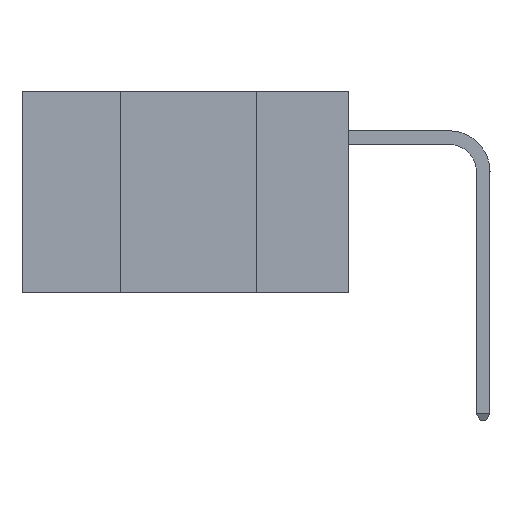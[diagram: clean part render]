
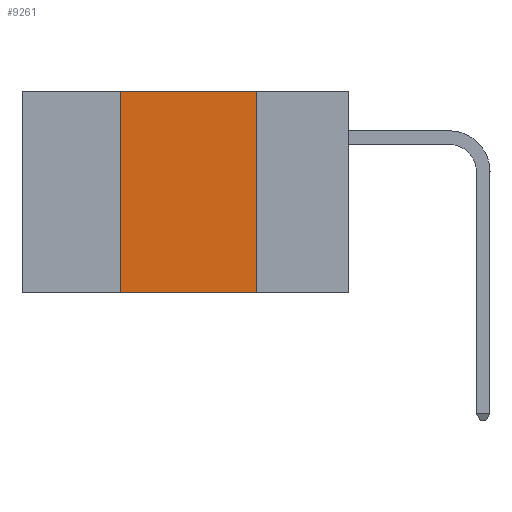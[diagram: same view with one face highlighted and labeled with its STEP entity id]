
A CAD part, left-side view. The second image highlights one B-rep face of the part: STEP entity #9261.
In plain terms, the highlighted planar face has unit normal (-1, 0, 0).
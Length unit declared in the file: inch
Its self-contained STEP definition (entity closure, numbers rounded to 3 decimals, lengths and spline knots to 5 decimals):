
#156 = CARTESIAN_POINT ( 'NONE',  ( 0., 0.6, 0. ) ) ;
#474 = EDGE_CURVE ( 'NONE', #7572, #5776, #1780, .T. ) ;
#669 = DIRECTION ( 'NONE',  ( 0., 0., -1. ) ) ;
#790 = FACE_OUTER_BOUND ( 'NONE', #6892, .T. ) ;
#1160 = CARTESIAN_POINT ( 'NONE',  ( 0., 0.42, 0. ) ) ;
#1184 = VECTOR ( 'NONE', #4738, 39.37008 ) ;
#1338 = DIRECTION ( 'NONE',  ( 0., 0., 1. ) ) ;
#1687 = VERTEX_POINT ( 'NONE', #3601 ) ;
#1709 = DIRECTION ( 'NONE',  ( 1., 0., 0. ) ) ;
#1780 = LINE ( 'NONE', #2579, #9054 ) ;
#1978 = CARTESIAN_POINT ( 'NONE',  ( 0., 0.17, -0.37 ) ) ;
#2056 = ORIENTED_EDGE ( 'NONE', *, *, #474, .T. ) ;
#2579 = CARTESIAN_POINT ( 'NONE',  ( 0., 0.6, -0.37 ) ) ;
#2707 = VECTOR ( 'NONE', #669, 39.37008 ) ;
#3147 = ORIENTED_EDGE ( 'NONE', *, *, #9012, .F. ) ;
#3256 = PLANE ( 'NONE',  #7125 ) ;
#3285 = CARTESIAN_POINT ( 'NONE',  ( 0., 0.6, 0. ) ) ;
#3353 = DIRECTION ( 'NONE',  ( 0., -1., 0. ) ) ;
#3601 = CARTESIAN_POINT ( 'NONE',  ( 0., 0.17, 0. ) ) ;
#3950 = EDGE_CURVE ( 'NONE', #9979, #1687, #5612, .T. ) ;
#4259 = ORIENTED_EDGE ( 'NONE', *, *, #3950, .F. ) ;
#4738 = DIRECTION ( 'NONE',  ( 0., -1., 0. ) ) ;
#5068 = DIRECTION ( 'NONE',  ( 0., 0., -1. ) ) ;
#5564 = CARTESIAN_POINT ( 'NONE',  ( 0., 0.42, 0. ) ) ;
#5612 = LINE ( 'NONE', #156, #1184 ) ;
#5776 = VERTEX_POINT ( 'NONE', #1978 ) ;
#6327 = VECTOR ( 'NONE', #1338, 39.37008 ) ;
#6350 = EDGE_CURVE ( 'NONE', #7572, #9979, #7912, .T. ) ;
#6700 = CARTESIAN_POINT ( 'NONE',  ( 0., 0.42, -0.37 ) ) ;
#6892 = EDGE_LOOP ( 'NONE', ( #3147, #4259, #7987, #2056 ) ) ;
#7002 = CARTESIAN_POINT ( 'NONE',  ( 0., 0.17, 0. ) ) ;
#7125 = AXIS2_PLACEMENT_3D ( 'NONE', #3285, #1709, #5068 ) ;
#7572 = VERTEX_POINT ( 'NONE', #6700 ) ;
#7912 = LINE ( 'NONE', #5564, #6327 ) ;
#7987 = ORIENTED_EDGE ( 'NONE', *, *, #6350, .F. ) ;
#9012 = EDGE_CURVE ( 'NONE', #1687, #5776, #9815, .T. ) ;
#9054 = VECTOR ( 'NONE', #3353, 39.37008 ) ;
#9261 = ADVANCED_FACE ( 'NONE', ( #790 ), #3256, .F. ) ;
#9815 = LINE ( 'NONE', #7002, #2707 ) ;
#9979 = VERTEX_POINT ( 'NONE', #1160 ) ;
